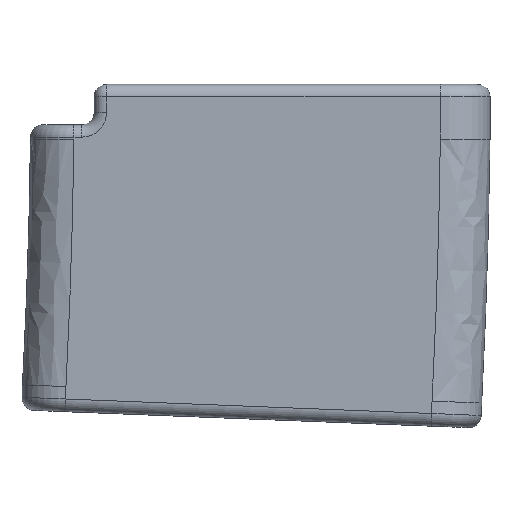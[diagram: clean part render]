
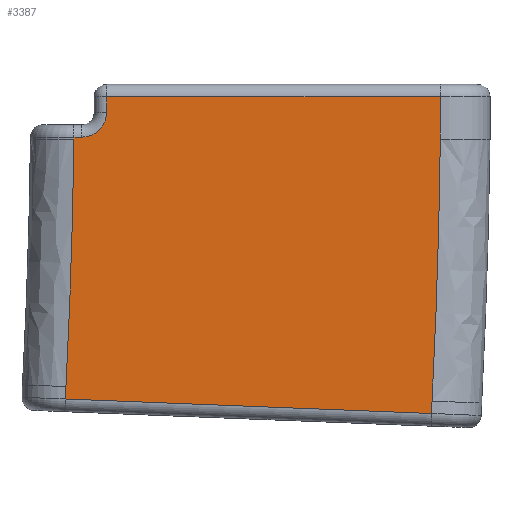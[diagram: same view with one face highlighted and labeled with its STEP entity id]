
A CAD part, top view. The second image highlights one B-rep face of the part: STEP entity #3387.
In plain terms, the highlighted planar face has unit normal (0, 0, 1).
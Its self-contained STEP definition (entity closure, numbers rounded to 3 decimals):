
#94=PLANE('',#3834);
#248=LINE('',#6307,#458);
#259=LINE('',#6338,#469);
#275=LINE('',#6379,#485);
#277=LINE('',#6392,#487);
#279=LINE('',#6400,#489);
#298=LINE('',#6475,#508);
#319=LINE('',#6693,#529);
#322=LINE('',#6699,#532);
#458=VECTOR('',#4552,10.);
#469=VECTOR('',#4579,10.);
#485=VECTOR('',#4633,10.);
#487=VECTOR('',#4649,10.);
#489=VECTOR('',#4657,10.);
#508=VECTOR('',#4748,10.);
#529=VECTOR('',#4883,10.);
#532=VECTOR('',#4892,10.);
#844=FACE_OUTER_BOUND('',#1062,.T.);
#1062=EDGE_LOOP('',(#3107,#3108,#3109,#3110,#3111,#3112,#3113,#3114,#3115,
#3116,#3117));
#1305=CIRCLE('',#3733,4.);
#1348=CIRCLE('',#3805,1007.545);
#1350=CIRCLE('',#3807,1066.541);
#1579=VERTEX_POINT('',#6277);
#1586=VERTEX_POINT('',#6303);
#1598=VERTEX_POINT('',#6337);
#1604=VERTEX_POINT('',#6377);
#1605=VERTEX_POINT('',#6383);
#1607=VERTEX_POINT('',#6387);
#1608=VERTEX_POINT('',#6391);
#1611=VERTEX_POINT('',#6399);
#1631=VERTEX_POINT('',#6473);
#1640=VERTEX_POINT('',#6612);
#1642=VERTEX_POINT('',#6625);
#2005=EDGE_CURVE('',#1586,#1579,#248,.T.);
#2020=EDGE_CURVE('',#1598,#1579,#259,.T.);
#2041=EDGE_CURVE('',#1604,#1586,#275,.T.);
#2046=EDGE_CURVE('',#1607,#1605,#1305,.T.);
#2047=EDGE_CURVE('',#1605,#1608,#277,.T.);
#2051=EDGE_CURVE('',#1608,#1611,#279,.T.);
#2090=EDGE_CURVE('',#1631,#1607,#298,.T.);
#2118=EDGE_CURVE('',#1640,#1598,#1348,.T.);
#2120=EDGE_CURVE('',#1642,#1604,#1350,.T.);
#2145=EDGE_CURVE('',#1631,#1640,#319,.T.);
#2148=EDGE_CURVE('',#1642,#1611,#322,.T.);
#3107=ORIENTED_EDGE('',*,*,#2005,.F.);
#3108=ORIENTED_EDGE('',*,*,#2041,.F.);
#3109=ORIENTED_EDGE('',*,*,#2120,.F.);
#3110=ORIENTED_EDGE('',*,*,#2148,.T.);
#3111=ORIENTED_EDGE('',*,*,#2051,.F.);
#3112=ORIENTED_EDGE('',*,*,#2047,.F.);
#3113=ORIENTED_EDGE('',*,*,#2046,.F.);
#3114=ORIENTED_EDGE('',*,*,#2090,.F.);
#3115=ORIENTED_EDGE('',*,*,#2145,.T.);
#3116=ORIENTED_EDGE('',*,*,#2118,.T.);
#3117=ORIENTED_EDGE('',*,*,#2020,.T.);
#3387=ADVANCED_FACE('',(#844),#94,.T.);
#3733=AXIS2_PLACEMENT_3D('',#6389,#4645,#4646);
#3805=AXIS2_PLACEMENT_3D('',#6614,#4816,#4817);
#3807=AXIS2_PLACEMENT_3D('',#6627,#4820,#4821);
#3834=AXIS2_PLACEMENT_3D('',#6700,#4893,#4894);
#4552=DIRECTION('',(-0.999,0.04,0.));
#4579=DIRECTION('',(-0.04,-0.999,0.));
#4633=DIRECTION('',(-0.04,-0.999,0.));
#4645=DIRECTION('center_axis',(0.,0.,1.));
#4646=DIRECTION('ref_axis',(0.487,-0.873,0.));
#4649=DIRECTION('',(0.,1.,0.));
#4657=DIRECTION('',(1.,0.,0.));
#4748=DIRECTION('',(1.,0.,0.));
#4816=DIRECTION('center_axis',(0.,0.,-1.));
#4817=DIRECTION('ref_axis',(1.,-0.013,0.));
#4820=DIRECTION('center_axis',(0.,0.,-1.));
#4821=DIRECTION('ref_axis',(1.,-0.012,0.));
#4883=DIRECTION('',(0.,-1.,0.));
#4892=DIRECTION('',(0.,1.,0.));
#4893=DIRECTION('center_axis',(0.,0.,1.));
#4894=DIRECTION('ref_axis',(1.,0.,0.));
#6277=CARTESIAN_POINT('',(-35.618,-44.16,14.95));
#6303=CARTESIAN_POINT('',(23.336,-46.495,14.95));
#6307=CARTESIAN_POINT('',(-19.277,-44.807,14.95));
#6337=CARTESIAN_POINT('',(-35.539,-42.161,14.95));
#6338=CARTESIAN_POINT('',(-35.539,-42.161,14.95));
#6377=CARTESIAN_POINT('',(23.415,-44.496,14.95));
#6379=CARTESIAN_POINT('',(23.415,-44.496,14.95));
#6383=CARTESIAN_POINT('',(-29.,2.,14.95));
#6387=CARTESIAN_POINT('',(-33.,-2.,14.95));
#6389=CARTESIAN_POINT('Origin',(-33.,2.,14.95));
#6391=CARTESIAN_POINT('',(-29.,4.5,14.95));
#6392=CARTESIAN_POINT('',(-29.,-1.15,14.95));
#6399=CARTESIAN_POINT('',(24.75,4.5,14.95));
#6400=CARTESIAN_POINT('',(-15.625,4.5,14.95));
#6473=CARTESIAN_POINT('',(-34.25,-2.,14.95));
#6475=CARTESIAN_POINT('',(-16.875,-2.,14.95));
#6612=CARTESIAN_POINT('',(-34.25,-2.3,14.95));
#6614=CARTESIAN_POINT('Origin',(-1041.716,10.329,14.95));
#6625=CARTESIAN_POINT('',(24.75,-2.3,14.95));
#6627=CARTESIAN_POINT('Origin',(-1041.716,10.329,14.95));
#6693=CARTESIAN_POINT('',(-34.25,0.,14.95));
#6699=CARTESIAN_POINT('',(24.75,-2.3,14.95));
#6700=CARTESIAN_POINT('Origin',(-31.25,-2.3,14.95));
